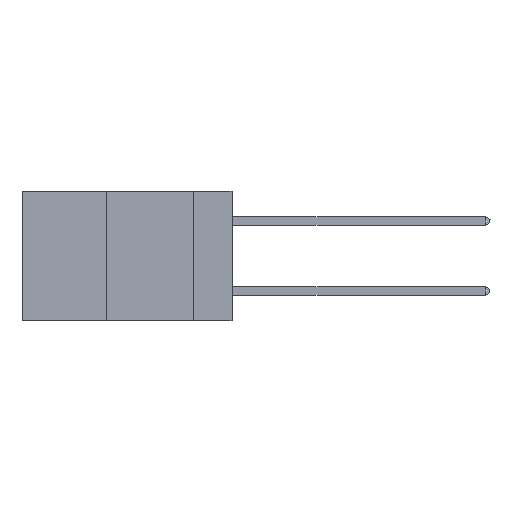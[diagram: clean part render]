
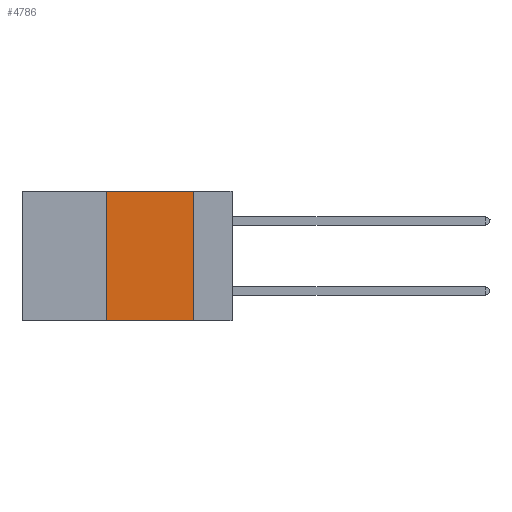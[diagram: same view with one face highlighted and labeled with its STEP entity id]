
A CAD part, left-side view. The second image highlights one B-rep face of the part: STEP entity #4786.
In plain terms, the highlighted planar face has unit normal (-1, 0, 0).
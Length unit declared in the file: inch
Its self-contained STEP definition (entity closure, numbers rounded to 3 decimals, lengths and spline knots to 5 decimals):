
#237 = ORIENTED_EDGE ( 'NONE', *, *, #5828, .F. ) ;
#308 = VECTOR ( 'NONE', #3838, 39.37008 ) ;
#1112 = DIRECTION ( 'NONE',  ( 0., 0., -1. ) ) ;
#1351 = CARTESIAN_POINT ( 'NONE',  ( 0., 0.36, 0. ) ) ;
#2089 = VERTEX_POINT ( 'NONE', #7203 ) ;
#2133 = AXIS2_PLACEMENT_3D ( 'NONE', #3519, #14684, #14376 ) ;
#3519 = CARTESIAN_POINT ( 'NONE',  ( 0., 0.6, 0. ) ) ;
#3838 = DIRECTION ( 'NONE',  ( 0., 0., 1. ) ) ;
#4634 = FACE_OUTER_BOUND ( 'NONE', #8138, .T. ) ;
#4786 = ADVANCED_FACE ( 'NONE', ( #4634 ), #15659, .F. ) ;
#5492 = DIRECTION ( 'NONE',  ( 0., -1., 0. ) ) ;
#5740 = EDGE_CURVE ( 'NONE', #15212, #2089, #13422, .T. ) ;
#5828 = EDGE_CURVE ( 'NONE', #14744, #7547, #12523, .T. ) ;
#6779 = LINE ( 'NONE', #6932, #13084 ) ;
#6932 = CARTESIAN_POINT ( 'NONE',  ( 0., 0.6, -0.37 ) ) ;
#7203 = CARTESIAN_POINT ( 'NONE',  ( 0., 0.11, -0.37 ) ) ;
#7244 = CARTESIAN_POINT ( 'NONE',  ( 0., 0.11, 0. ) ) ;
#7248 = CARTESIAN_POINT ( 'NONE',  ( 0., 0.6, 0. ) ) ;
#7547 = VERTEX_POINT ( 'NONE', #12259 ) ;
#8138 = EDGE_LOOP ( 'NONE', ( #14615, #10486, #237, #14123 ) ) ;
#8446 = CARTESIAN_POINT ( 'NONE',  ( 0., 0.11, 0. ) ) ;
#10486 = ORIENTED_EDGE ( 'NONE', *, *, #10782, .F. ) ;
#10782 = EDGE_CURVE ( 'NONE', #7547, #15212, #14562, .T. ) ;
#11231 = VECTOR ( 'NONE', #14637, 39.37008 ) ;
#11632 = VECTOR ( 'NONE', #1112, 39.37008 ) ;
#12259 = CARTESIAN_POINT ( 'NONE',  ( 0., 0.36, 0. ) ) ;
#12523 = LINE ( 'NONE', #1351, #308 ) ;
#13084 = VECTOR ( 'NONE', #5492, 39.37008 ) ;
#13422 = LINE ( 'NONE', #7244, #11632 ) ;
#13687 = EDGE_CURVE ( 'NONE', #14744, #2089, #6779, .T. ) ;
#14123 = ORIENTED_EDGE ( 'NONE', *, *, #13687, .T. ) ;
#14376 = DIRECTION ( 'NONE',  ( 0., 0., -1. ) ) ;
#14562 = LINE ( 'NONE', #7248, #11231 ) ;
#14615 = ORIENTED_EDGE ( 'NONE', *, *, #5740, .F. ) ;
#14637 = DIRECTION ( 'NONE',  ( 0., -1., 0. ) ) ;
#14684 = DIRECTION ( 'NONE',  ( 1., 0., 0. ) ) ;
#14744 = VERTEX_POINT ( 'NONE', #15292 ) ;
#15212 = VERTEX_POINT ( 'NONE', #8446 ) ;
#15292 = CARTESIAN_POINT ( 'NONE',  ( 0., 0.36, -0.37 ) ) ;
#15659 = PLANE ( 'NONE',  #2133 ) ;
